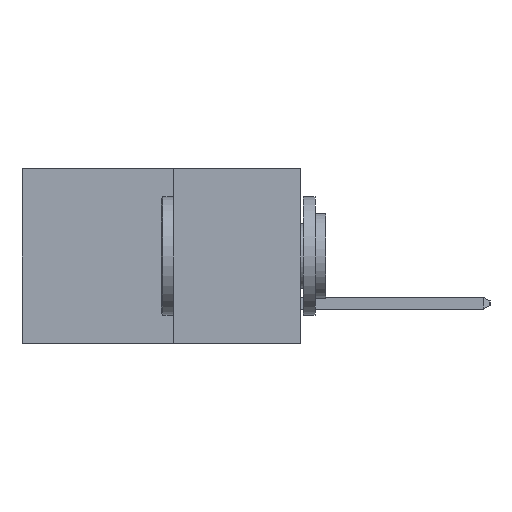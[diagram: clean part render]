
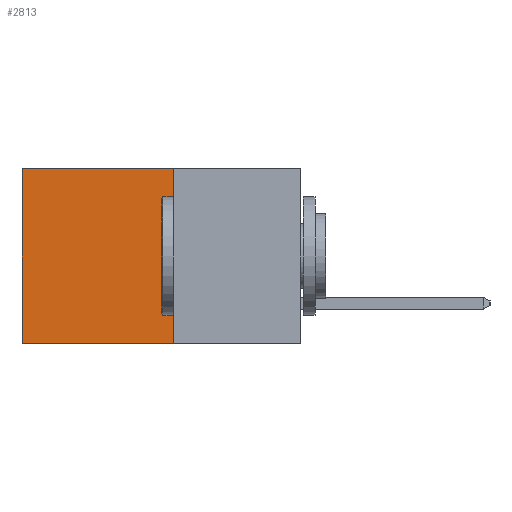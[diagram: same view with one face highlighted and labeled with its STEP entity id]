
A CAD part, left-side view. The second image highlights one B-rep face of the part: STEP entity #2813.
In plain terms, the highlighted planar face has unit normal (-1, 0, 0).
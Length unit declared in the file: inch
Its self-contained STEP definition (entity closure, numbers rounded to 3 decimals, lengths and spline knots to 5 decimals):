
#192 = DIRECTION ( 'NONE',  ( 0., 0., -1. ) ) ;
#611 = FACE_OUTER_BOUND ( 'NONE', #1701, .T. ) ;
#1015 = EDGE_CURVE ( 'NONE', #2848, #5414, #1536, .T. ) ;
#1302 = PLANE ( 'NONE',  #6340 ) ;
#1367 = EDGE_CURVE ( 'NONE', #2848, #3029, #8804, .T. ) ;
#1536 = LINE ( 'NONE', #1782, #3959 ) ;
#1701 = EDGE_LOOP ( 'NONE', ( #4634, #5149, #7223, #2908 ) ) ;
#1782 = CARTESIAN_POINT ( 'NONE',  ( 0.277, 0.27, 0. ) ) ;
#1837 = CARTESIAN_POINT ( 'NONE',  ( 0.277, 0.27, -0.37 ) ) ;
#1908 = DIRECTION ( 'NONE',  ( 0., 1., 0. ) ) ;
#1914 = LINE ( 'NONE', #8186, #10047 ) ;
#2274 = CARTESIAN_POINT ( 'NONE',  ( 0.277, 0.27, -0.37 ) ) ;
#2813 = ADVANCED_FACE ( 'NONE', ( #611 ), #1302, .F. ) ;
#2848 = VERTEX_POINT ( 'NONE', #8985 ) ;
#2908 = ORIENTED_EDGE ( 'NONE', *, *, #1015, .T. ) ;
#3029 = VERTEX_POINT ( 'NONE', #1837 ) ;
#3959 = VECTOR ( 'NONE', #1908, 39.37008 ) ;
#3966 = EDGE_CURVE ( 'NONE', #5414, #8365, #1914, .T. ) ;
#4365 = CARTESIAN_POINT ( 'NONE',  ( 0.277, 0.59, -0.37 ) ) ;
#4634 = ORIENTED_EDGE ( 'NONE', *, *, #3966, .T. ) ;
#4682 = VECTOR ( 'NONE', #9840, 39.37008 ) ;
#5149 = ORIENTED_EDGE ( 'NONE', *, *, #7798, .F. ) ;
#5285 = DIRECTION ( 'NONE',  ( 0., 1., 0. ) ) ;
#5377 = LINE ( 'NONE', #9119, #8992 ) ;
#5414 = VERTEX_POINT ( 'NONE', #9616 ) ;
#5891 = CARTESIAN_POINT ( 'NONE',  ( 0.277, 0.27, -0.37 ) ) ;
#6340 = AXIS2_PLACEMENT_3D ( 'NONE', #2274, #8879, #192 ) ;
#7223 = ORIENTED_EDGE ( 'NONE', *, *, #1367, .F. ) ;
#7798 = EDGE_CURVE ( 'NONE', #3029, #8365, #5377, .T. ) ;
#8070 = DIRECTION ( 'NONE',  ( 0., 0., -1. ) ) ;
#8186 = CARTESIAN_POINT ( 'NONE',  ( 0.277, 0.59, -0.37 ) ) ;
#8365 = VERTEX_POINT ( 'NONE', #4365 ) ;
#8804 = LINE ( 'NONE', #5891, #4682 ) ;
#8879 = DIRECTION ( 'NONE',  ( 1., 0., 0. ) ) ;
#8985 = CARTESIAN_POINT ( 'NONE',  ( 0.277, 0.27, 0. ) ) ;
#8992 = VECTOR ( 'NONE', #5285, 39.37008 ) ;
#9119 = CARTESIAN_POINT ( 'NONE',  ( 0.277, 0.27, -0.37 ) ) ;
#9616 = CARTESIAN_POINT ( 'NONE',  ( 0.277, 0.59, 0. ) ) ;
#9840 = DIRECTION ( 'NONE',  ( 0., 0., -1. ) ) ;
#10047 = VECTOR ( 'NONE', #8070, 39.37008 ) ;
